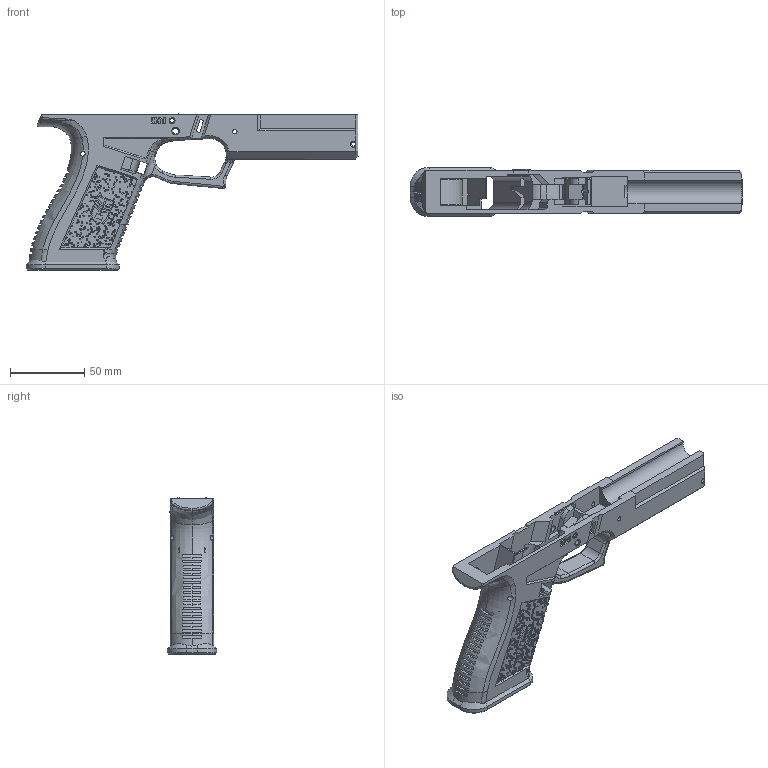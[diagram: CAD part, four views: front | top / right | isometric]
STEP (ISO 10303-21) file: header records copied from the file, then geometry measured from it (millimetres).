
FILE_DESCRIPTION(/* description */ (''),/* implementation_level */ '2;1');
FILE_NAME(/* name */ 'DD17.2 GXL C34.step',/* time_stamp */ '2022-07-31T11:02:39-05:00',/* author */ (''),/* organization */ (''),/* preprocessor_version */ 'ST-DEVELOPER v19',/* originating_system */ 'Autodesk Translation Framework v11.7.0.108',/* authorisation */ '');
FILE_SCHEMA (('AUTOMOTIVE_DESIGN { 1 0 10303 214 3 1 1 }'));
Products named in the file (1): DD17.2 SDI GXL Competition
Bounding box: 223.95 x 33.23 x 105.56 mm (x, y, z)
Volume: 132788 mm3; surface area: 60256.2 mm2
Topology: 1 solids, 2 shells, 3246 faces, 8409 edges, 5541 vertices
Faces by surface type: bspline 2237, plane 932, cylinder 62, torus 9, cone 6
Full cylindrical faces by diameter (mm): 1.933 x1, 3 x6, 3.2 x2, 3.5 x1, 4.1 x2, 14 x1
Entity records: 132220 total; most frequent: CARTESIAN_POINT 74726, ORIENTED_EDGE 16806, EDGE_CURVE 8403, DIRECTION 5720, VERTEX_POINT 5541, EDGE_LOOP 3662, LINE 3304, VECTOR 3304
